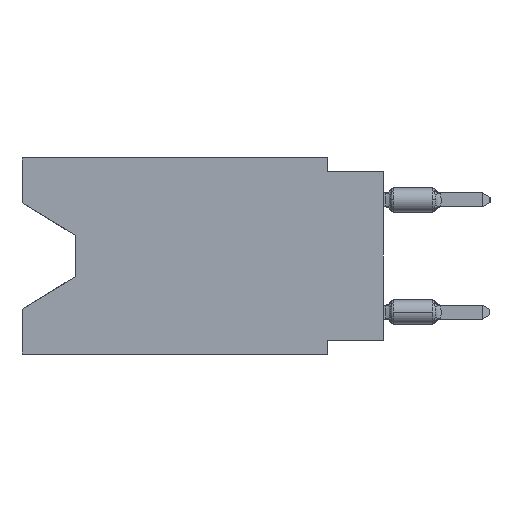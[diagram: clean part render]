
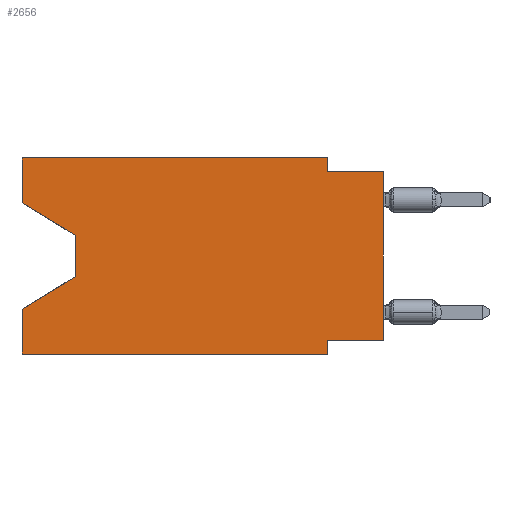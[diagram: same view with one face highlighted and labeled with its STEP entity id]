
A CAD part, left-side view. The second image highlights one B-rep face of the part: STEP entity #2656.
In plain terms, the highlighted planar face has unit normal (-1, 0, 0).
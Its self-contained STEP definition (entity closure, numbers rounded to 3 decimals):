
#69 = VECTOR ( 'NONE', #16623, 1000. ) ;
#1122 = CARTESIAN_POINT ( 'NONE',  ( 0., 0., -0.635 ) ) ;
#1282 = VERTEX_POINT ( 'NONE', #23671 ) ;
#1563 = EDGE_CURVE ( 'NONE', #48799, #1961, #32340, .T. ) ;
#1573 = EDGE_CURVE ( 'NONE', #36298, #11865, #5367, .T. ) ;
#1680 = VECTOR ( 'NONE', #24138, 1000. ) ;
#1961 = VERTEX_POINT ( 'NONE', #21733 ) ;
#2104 = CARTESIAN_POINT ( 'NONE',  ( 0., 16.383, -8.89 ) ) ;
#2446 = DIRECTION ( 'NONE',  ( 0., -1., 0. ) ) ;
#2448 = VERTEX_POINT ( 'NONE', #31396 ) ;
#2656 = ADVANCED_FACE ( 'NONE', ( #48278 ), #40292, .F. ) ;
#3725 = DIRECTION ( 'NONE',  ( 0., -0.855, -0.519 ) ) ;
#4320 = VECTOR ( 'NONE', #42603, 1000. ) ;
#4529 = LINE ( 'NONE', #43014, #41562 ) ;
#4856 = LINE ( 'NONE', #27607, #37321 ) ;
#4865 = CARTESIAN_POINT ( 'NONE',  ( 0., 16.383, -8.89 ) ) ;
#5367 = LINE ( 'NONE', #1122, #69 ) ;
#5816 = DIRECTION ( 'NONE',  ( 0., 0., -1. ) ) ;
#6232 = LINE ( 'NONE', #32472, #12095 ) ;
#8472 = VERTEX_POINT ( 'NONE', #17912 ) ;
#9029 = DIRECTION ( 'NONE',  ( 0., 0., 1. ) ) ;
#9523 = EDGE_CURVE ( 'NONE', #11927, #41293, #4529, .T. ) ;
#10442 = LINE ( 'NONE', #48910, #18771 ) ;
#11120 = ORIENTED_EDGE ( 'NONE', *, *, #1573, .F. ) ;
#11532 = EDGE_CURVE ( 'NONE', #2448, #26064, #17047, .T. ) ;
#11725 = CARTESIAN_POINT ( 'NONE',  ( 0., 2.54, 0. ) ) ;
#11865 = VERTEX_POINT ( 'NONE', #43234 ) ;
#11927 = VERTEX_POINT ( 'NONE', #35724 ) ;
#12095 = VECTOR ( 'NONE', #21487, 1000. ) ;
#12397 = CARTESIAN_POINT ( 'NONE',  ( 0., 16.383, 0. ) ) ;
#13298 = CARTESIAN_POINT ( 'NONE',  ( 0., 16.383, 0. ) ) ;
#14388 = VERTEX_POINT ( 'NONE', #11725 ) ;
#14751 = CARTESIAN_POINT ( 'NONE',  ( 0., 2.54, -0.635 ) ) ;
#14923 = DIRECTION ( 'NONE',  ( 0., 0., -1. ) ) ;
#15236 = LINE ( 'NONE', #22728, #18914 ) ;
#15560 = ORIENTED_EDGE ( 'NONE', *, *, #1563, .T. ) ;
#16623 = DIRECTION ( 'NONE',  ( 0., -1., 0. ) ) ;
#17047 = LINE ( 'NONE', #13298, #38700 ) ;
#17595 = EDGE_CURVE ( 'NONE', #1961, #1282, #45091, .T. ) ;
#17912 = CARTESIAN_POINT ( 'NONE',  ( 0., 2.54, -8.89 ) ) ;
#18240 = ORIENTED_EDGE ( 'NONE', *, *, #28192, .T. ) ;
#18324 = ORIENTED_EDGE ( 'NONE', *, *, #11532, .F. ) ;
#18771 = VECTOR ( 'NONE', #2446, 1000. ) ;
#18914 = VECTOR ( 'NONE', #3725, 1000. ) ;
#19125 = EDGE_CURVE ( 'NONE', #32767, #1282, #25004, .T. ) ;
#20884 = AXIS2_PLACEMENT_3D ( 'NONE', #12397, #39380, #5816 ) ;
#21487 = DIRECTION ( 'NONE',  ( 0., 0., 1. ) ) ;
#21733 = CARTESIAN_POINT ( 'NONE',  ( 0., 13.97, -5.385 ) ) ;
#22274 = EDGE_CURVE ( 'NONE', #11927, #11865, #6232, .T. ) ;
#22608 = CARTESIAN_POINT ( 'NONE',  ( 0., 13.97, -5.385 ) ) ;
#22728 = CARTESIAN_POINT ( 'NONE',  ( 0., 16.383, -2.038 ) ) ;
#23671 = CARTESIAN_POINT ( 'NONE',  ( 0., 16.383, -6.852 ) ) ;
#24138 = DIRECTION ( 'NONE',  ( 0., 0., -1. ) ) ;
#24785 = ORIENTED_EDGE ( 'NONE', *, *, #17595, .T. ) ;
#24943 = EDGE_CURVE ( 'NONE', #2448, #48799, #15236, .T. ) ;
#25004 = LINE ( 'NONE', #40232, #46106 ) ;
#25365 = EDGE_CURVE ( 'NONE', #41293, #8472, #29432, .T. ) ;
#26064 = VERTEX_POINT ( 'NONE', #27485 ) ;
#26313 = EDGE_CURVE ( 'NONE', #26064, #14388, #10442, .T. ) ;
#26408 = ORIENTED_EDGE ( 'NONE', *, *, #26313, .F. ) ;
#27485 = CARTESIAN_POINT ( 'NONE',  ( 0., 16.383, 0. ) ) ;
#27607 = CARTESIAN_POINT ( 'NONE',  ( 0., 2.54, 0. ) ) ;
#28118 = LINE ( 'NONE', #4865, #4320 ) ;
#28192 = EDGE_CURVE ( 'NONE', #32767, #8472, #28118, .T. ) ;
#28517 = VECTOR ( 'NONE', #33838, 1000. ) ;
#28543 = DIRECTION ( 'NONE',  ( 0., 0., 1. ) ) ;
#29110 = ORIENTED_EDGE ( 'NONE', *, *, #19125, .F. ) ;
#29432 = LINE ( 'NONE', #37153, #45169 ) ;
#29854 = ORIENTED_EDGE ( 'NONE', *, *, #25365, .F. ) ;
#30957 = CARTESIAN_POINT ( 'NONE',  ( 0., 13.97, -3.505 ) ) ;
#31396 = CARTESIAN_POINT ( 'NONE',  ( 0., 16.383, -2.038 ) ) ;
#32340 = LINE ( 'NONE', #39601, #1680 ) ;
#32472 = CARTESIAN_POINT ( 'NONE',  ( 0., 0., 0. ) ) ;
#32767 = VERTEX_POINT ( 'NONE', #2104 ) ;
#33838 = DIRECTION ( 'NONE',  ( 0., 0.855, -0.519 ) ) ;
#34619 = EDGE_CURVE ( 'NONE', #14388, #36298, #4856, .T. ) ;
#35724 = CARTESIAN_POINT ( 'NONE',  ( 0., 0., -8.255 ) ) ;
#36298 = VERTEX_POINT ( 'NONE', #14751 ) ;
#37153 = CARTESIAN_POINT ( 'NONE',  ( 0., 2.54, -8.89 ) ) ;
#37321 = VECTOR ( 'NONE', #39096, 1000. ) ;
#37365 = ORIENTED_EDGE ( 'NONE', *, *, #22274, .T. ) ;
#38700 = VECTOR ( 'NONE', #28543, 1000. ) ;
#39096 = DIRECTION ( 'NONE',  ( 0., 0., -1. ) ) ;
#39261 = DIRECTION ( 'NONE',  ( 0., 1., 0. ) ) ;
#39380 = DIRECTION ( 'NONE',  ( 1., 0., 0. ) ) ;
#39601 = CARTESIAN_POINT ( 'NONE',  ( 0., 13.97, -3.505 ) ) ;
#40232 = CARTESIAN_POINT ( 'NONE',  ( 0., 16.383, 0. ) ) ;
#40292 = PLANE ( 'NONE',  #20884 ) ;
#41293 = VERTEX_POINT ( 'NONE', #47312 ) ;
#41562 = VECTOR ( 'NONE', #39261, 1000. ) ;
#41894 = ORIENTED_EDGE ( 'NONE', *, *, #34619, .F. ) ;
#41981 = ORIENTED_EDGE ( 'NONE', *, *, #24943, .T. ) ;
#42336 = ORIENTED_EDGE ( 'NONE', *, *, #9523, .F. ) ;
#42603 = DIRECTION ( 'NONE',  ( 0., -1., 0. ) ) ;
#43014 = CARTESIAN_POINT ( 'NONE',  ( 0., 0., -8.255 ) ) ;
#43234 = CARTESIAN_POINT ( 'NONE',  ( 0., 0., -0.635 ) ) ;
#43700 = EDGE_LOOP ( 'NONE', ( #41981, #15560, #24785, #29110, #18240, #29854, #42336, #37365, #11120, #41894, #26408, #18324 ) ) ;
#45091 = LINE ( 'NONE', #22608, #28517 ) ;
#45169 = VECTOR ( 'NONE', #14923, 1000. ) ;
#46106 = VECTOR ( 'NONE', #9029, 1000. ) ;
#47312 = CARTESIAN_POINT ( 'NONE',  ( 0., 2.54, -8.255 ) ) ;
#48278 = FACE_OUTER_BOUND ( 'NONE', #43700, .T. ) ;
#48799 = VERTEX_POINT ( 'NONE', #30957 ) ;
#48910 = CARTESIAN_POINT ( 'NONE',  ( 0., 16.383, 0. ) ) ;
